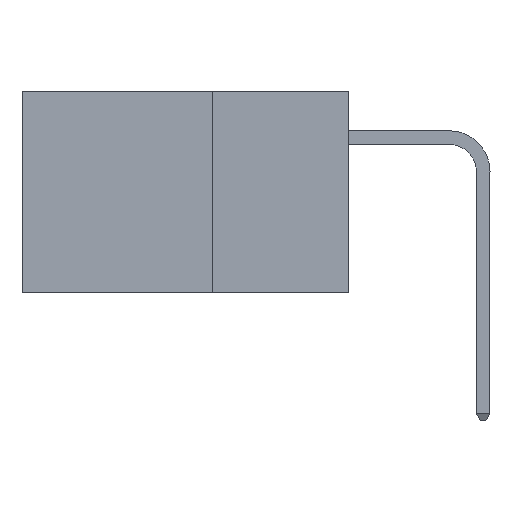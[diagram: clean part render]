
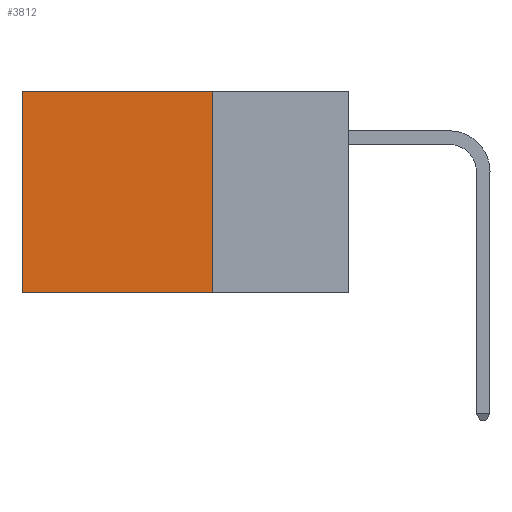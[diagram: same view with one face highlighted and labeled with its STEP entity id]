
A CAD part, left-side view. The second image highlights one B-rep face of the part: STEP entity #3812.
In plain terms, the highlighted planar face has unit normal (-1, 0, 0).
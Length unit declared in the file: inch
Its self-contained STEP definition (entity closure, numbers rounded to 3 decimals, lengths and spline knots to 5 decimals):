
#964 = VERTEX_POINT ( 'NONE', #1764 ) ;
#1079 = VERTEX_POINT ( 'NONE', #3857 ) ;
#1167 = VECTOR ( 'NONE', #4074, 39.37008 ) ;
#1261 = LINE ( 'NONE', #8357, #5193 ) ;
#1417 = LINE ( 'NONE', #14232, #5341 ) ;
#1764 = CARTESIAN_POINT ( 'NONE',  ( 0.2875, 0.25, -0.37 ) ) ;
#1769 = DIRECTION ( 'NONE',  ( 0., 0., -1. ) ) ;
#1840 = CARTESIAN_POINT ( 'NONE',  ( 0.2875, 0.25, -0.37 ) ) ;
#2082 = EDGE_CURVE ( 'NONE', #1079, #9380, #5614, .T. ) ;
#2335 = EDGE_CURVE ( 'NONE', #7776, #1079, #1417, .T. ) ;
#2772 = CARTESIAN_POINT ( 'NONE',  ( 0.2875, 0.6, -0.37 ) ) ;
#2816 = DIRECTION ( 'NONE',  ( 1., 0., 0. ) ) ;
#3575 = DIRECTION ( 'NONE',  ( 0., 1., 0. ) ) ;
#3812 = ADVANCED_FACE ( 'NONE', ( #7487 ), #8940, .F. ) ;
#3857 = CARTESIAN_POINT ( 'NONE',  ( 0.2875, 0.6, 0. ) ) ;
#4074 = DIRECTION ( 'NONE',  ( 0., 0., -1. ) ) ;
#5193 = VECTOR ( 'NONE', #9959, 39.37008 ) ;
#5341 = VECTOR ( 'NONE', #14002, 39.37008 ) ;
#5614 = LINE ( 'NONE', #6376, #1167 ) ;
#6376 = CARTESIAN_POINT ( 'NONE',  ( 0.2875, 0.6, 0. ) ) ;
#6675 = EDGE_LOOP ( 'NONE', ( #12354, #17524, #9991, #19942 ) ) ;
#7487 = FACE_OUTER_BOUND ( 'NONE', #6675, .T. ) ;
#7776 = VERTEX_POINT ( 'NONE', #19035 ) ;
#7829 = CARTESIAN_POINT ( 'NONE',  ( 0.2875, 0.25, 0. ) ) ;
#7897 = LINE ( 'NONE', #1840, #19849 ) ;
#8357 = CARTESIAN_POINT ( 'NONE',  ( 0.2875, 0.25, 0. ) ) ;
#8940 = PLANE ( 'NONE',  #10132 ) ;
#9380 = VERTEX_POINT ( 'NONE', #2772 ) ;
#9959 = DIRECTION ( 'NONE',  ( 0., 0., -1. ) ) ;
#9991 = ORIENTED_EDGE ( 'NONE', *, *, #18391, .F. ) ;
#10132 = AXIS2_PLACEMENT_3D ( 'NONE', #7829, #2816, #1769 ) ;
#12354 = ORIENTED_EDGE ( 'NONE', *, *, #2082, .T. ) ;
#14002 = DIRECTION ( 'NONE',  ( 0., 1., 0. ) ) ;
#14232 = CARTESIAN_POINT ( 'NONE',  ( 0.2875, 0.25, 0. ) ) ;
#15510 = EDGE_CURVE ( 'NONE', #964, #9380, #7897, .T. ) ;
#17524 = ORIENTED_EDGE ( 'NONE', *, *, #15510, .F. ) ;
#18391 = EDGE_CURVE ( 'NONE', #7776, #964, #1261, .T. ) ;
#19035 = CARTESIAN_POINT ( 'NONE',  ( 0.2875, 0.25, 0. ) ) ;
#19849 = VECTOR ( 'NONE', #3575, 39.37008 ) ;
#19942 = ORIENTED_EDGE ( 'NONE', *, *, #2335, .T. ) ;
